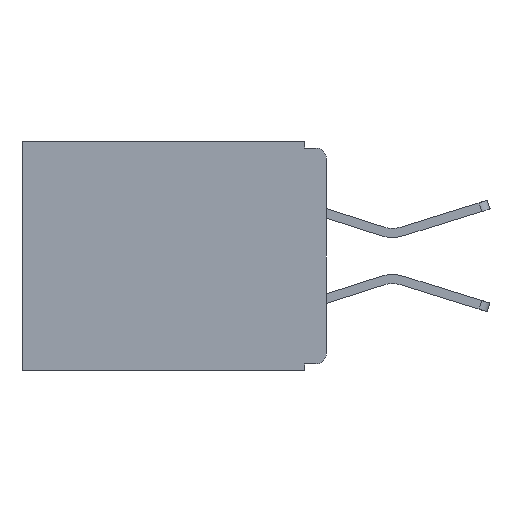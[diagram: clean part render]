
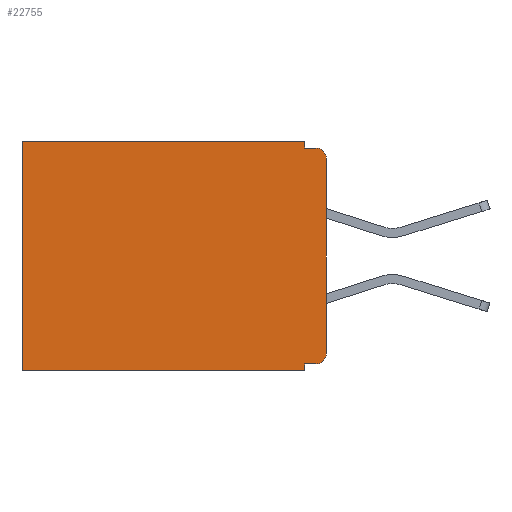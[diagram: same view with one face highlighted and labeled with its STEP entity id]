
A CAD part, left-side view. The second image highlights one B-rep face of the part: STEP entity #22755.
In plain terms, the highlighted planar face has unit normal (-1, 0, 0).
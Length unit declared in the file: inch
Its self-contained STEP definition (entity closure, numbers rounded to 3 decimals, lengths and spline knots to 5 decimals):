
#56 = DIRECTION ( 'NONE',  ( 0., 0., -1. ) ) ;
#751 = CARTESIAN_POINT ( 'NONE',  ( 0.3, 0.031, 0. ) ) ;
#821 = EDGE_CURVE ( 'NONE', #8801, #20920, #3724, .T. ) ;
#1290 = VECTOR ( 'NONE', #21838, 39.37008 ) ;
#1506 = CARTESIAN_POINT ( 'NONE',  ( 0.3, 0., -0.33 ) ) ;
#1670 = VERTEX_POINT ( 'NONE', #24347 ) ;
#1738 = ORIENTED_EDGE ( 'NONE', *, *, #821, .F. ) ;
#1746 = DIRECTION ( 'NONE',  ( 0., 1., 0. ) ) ;
#2813 = AXIS2_PLACEMENT_3D ( 'NONE', #21409, #6875, #23851 ) ;
#3084 = EDGE_CURVE ( 'NONE', #16561, #21481, #7012, .T. ) ;
#3701 = EDGE_CURVE ( 'NONE', #16561, #11639, #9135, .T. ) ;
#3724 = LINE ( 'NONE', #1506, #22340 ) ;
#3733 = AXIS2_PLACEMENT_3D ( 'NONE', #10005, #26946, #12452 ) ;
#3881 = EDGE_CURVE ( 'NONE', #24701, #9546, #11027, .T. ) ;
#4263 = VECTOR ( 'NONE', #21266, 39.37008 ) ;
#4775 = CARTESIAN_POINT ( 'NONE',  ( 0.3, 0.015, -0.01 ) ) ;
#4794 = DIRECTION ( 'NONE',  ( -1., 0., 0. ) ) ;
#5130 = DIRECTION ( 'NONE',  ( 0., 0., -1. ) ) ;
#5176 = CARTESIAN_POINT ( 'NONE',  ( 0.3, 0.015, -0.025 ) ) ;
#5452 = AXIS2_PLACEMENT_3D ( 'NONE', #5176, #4794, #5130 ) ;
#6452 = CARTESIAN_POINT ( 'NONE',  ( 0.3, 0., -0.01 ) ) ;
#6875 = DIRECTION ( 'NONE',  ( 1., 0., 0. ) ) ;
#7012 = LINE ( 'NONE', #27767, #1290 ) ;
#7642 = ORIENTED_EDGE ( 'NONE', *, *, #17653, .F. ) ;
#7737 = ORIENTED_EDGE ( 'NONE', *, *, #8612, .F. ) ;
#8404 = DIRECTION ( 'NONE',  ( 0., 0., -1. ) ) ;
#8612 = EDGE_CURVE ( 'NONE', #1670, #27343, #24377, .T. ) ;
#8801 = VERTEX_POINT ( 'NONE', #26831 ) ;
#9135 = CIRCLE ( 'NONE', #5452, 0.015 ) ;
#9546 = VERTEX_POINT ( 'NONE', #23696 ) ;
#10005 = CARTESIAN_POINT ( 'NONE',  ( 0.3, 0.015, -0.305 ) ) ;
#10094 = ORIENTED_EDGE ( 'NONE', *, *, #3881, .T. ) ;
#10481 = CARTESIAN_POINT ( 'NONE',  ( 0.3, 0., -0.025 ) ) ;
#10728 = EDGE_LOOP ( 'NONE', ( #20001, #21024, #25889, #7642, #10094, #12744, #1738, #27153, #7737, #17905 ) ) ;
#10966 = LINE ( 'NONE', #23849, #23121 ) ;
#11027 = LINE ( 'NONE', #26339, #17424 ) ;
#11639 = VERTEX_POINT ( 'NONE', #4775 ) ;
#12452 = DIRECTION ( 'NONE',  ( 0., 0., -1. ) ) ;
#12482 = LINE ( 'NONE', #29053, #24625 ) ;
#12744 = ORIENTED_EDGE ( 'NONE', *, *, #18483, .T. ) ;
#13766 = CIRCLE ( 'NONE', #3733, 0.015 ) ;
#13829 = CARTESIAN_POINT ( 'NONE',  ( 0.3, 0.031, -0.01 ) ) ;
#13938 = CARTESIAN_POINT ( 'NONE',  ( 0.3, 0., -0.32 ) ) ;
#14434 = EDGE_CURVE ( 'NONE', #27343, #8801, #12482, .T. ) ;
#15492 = VECTOR ( 'NONE', #23440, 39.37008 ) ;
#16561 = VERTEX_POINT ( 'NONE', #10481 ) ;
#16682 = LINE ( 'NONE', #30141, #28779 ) ;
#16813 = CARTESIAN_POINT ( 'NONE',  ( 0.3, 0.437, -0.33 ) ) ;
#17424 = VECTOR ( 'NONE', #26447, 39.37008 ) ;
#17653 = EDGE_CURVE ( 'NONE', #24701, #23320, #16682, .T. ) ;
#17905 = ORIENTED_EDGE ( 'NONE', *, *, #28636, .T. ) ;
#18317 = EDGE_CURVE ( 'NONE', #23320, #11639, #22746, .T. ) ;
#18483 = EDGE_CURVE ( 'NONE', #9546, #20920, #10966, .T. ) ;
#18992 = CARTESIAN_POINT ( 'NONE',  ( 0.3, 0., -0.305 ) ) ;
#20001 = ORIENTED_EDGE ( 'NONE', *, *, #3084, .F. ) ;
#20920 = VERTEX_POINT ( 'NONE', #16813 ) ;
#21024 = ORIENTED_EDGE ( 'NONE', *, *, #3701, .T. ) ;
#21266 = DIRECTION ( 'NONE',  ( 0., 1., 0. ) ) ;
#21409 = CARTESIAN_POINT ( 'NONE',  ( 0.3, 0., -0.33 ) ) ;
#21481 = VERTEX_POINT ( 'NONE', #18992 ) ;
#21838 = DIRECTION ( 'NONE',  ( 0., 0., -1. ) ) ;
#22340 = VECTOR ( 'NONE', #1746, 39.37008 ) ;
#22746 = LINE ( 'NONE', #6452, #15492 ) ;
#22755 = ADVANCED_FACE ( 'NONE', ( #25533 ), #30919, .F. ) ;
#23121 = VECTOR ( 'NONE', #24041, 39.37008 ) ;
#23320 = VERTEX_POINT ( 'NONE', #13829 ) ;
#23440 = DIRECTION ( 'NONE',  ( 0., -1., 0. ) ) ;
#23696 = CARTESIAN_POINT ( 'NONE',  ( 0.3, 0.437, 0. ) ) ;
#23849 = CARTESIAN_POINT ( 'NONE',  ( 0.3, 0.437, -0.33 ) ) ;
#23851 = DIRECTION ( 'NONE',  ( 0., 0., -1. ) ) ;
#23975 = CARTESIAN_POINT ( 'NONE',  ( 0.3, 0.031, -0.32 ) ) ;
#24041 = DIRECTION ( 'NONE',  ( 0., 0., -1. ) ) ;
#24347 = CARTESIAN_POINT ( 'NONE',  ( 0.3, 0.015, -0.32 ) ) ;
#24377 = LINE ( 'NONE', #13938, #4263 ) ;
#24625 = VECTOR ( 'NONE', #56, 39.37008 ) ;
#24701 = VERTEX_POINT ( 'NONE', #751 ) ;
#25533 = FACE_OUTER_BOUND ( 'NONE', #10728, .T. ) ;
#25889 = ORIENTED_EDGE ( 'NONE', *, *, #18317, .F. ) ;
#26339 = CARTESIAN_POINT ( 'NONE',  ( 0.3, 0., 0. ) ) ;
#26447 = DIRECTION ( 'NONE',  ( 0., 1., 0. ) ) ;
#26831 = CARTESIAN_POINT ( 'NONE',  ( 0.3, 0.031, -0.33 ) ) ;
#26946 = DIRECTION ( 'NONE',  ( -1., 0., 0. ) ) ;
#27153 = ORIENTED_EDGE ( 'NONE', *, *, #14434, .F. ) ;
#27343 = VERTEX_POINT ( 'NONE', #23975 ) ;
#27767 = CARTESIAN_POINT ( 'NONE',  ( 0.3, 0., -0.33 ) ) ;
#28636 = EDGE_CURVE ( 'NONE', #1670, #21481, #13766, .T. ) ;
#28779 = VECTOR ( 'NONE', #8404, 39.37008 ) ;
#29053 = CARTESIAN_POINT ( 'NONE',  ( 0.3, 0.031, -0.33 ) ) ;
#30141 = CARTESIAN_POINT ( 'NONE',  ( 0.3, 0.031, 0. ) ) ;
#30919 = PLANE ( 'NONE',  #2813 ) ;
